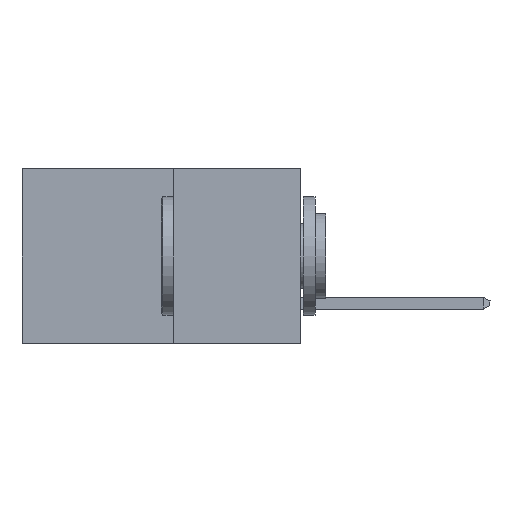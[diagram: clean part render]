
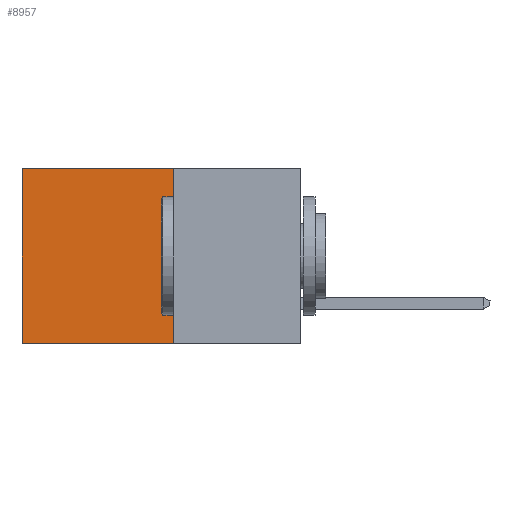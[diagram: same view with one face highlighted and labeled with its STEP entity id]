
A CAD part, left-side view. The second image highlights one B-rep face of the part: STEP entity #8957.
In plain terms, the highlighted planar face has unit normal (-1, 0, 0).
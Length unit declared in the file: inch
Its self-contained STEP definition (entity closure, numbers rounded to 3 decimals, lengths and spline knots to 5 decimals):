
#61 = DIRECTION ( 'NONE',  ( 0., 0., -1. ) ) ;
#277 = CARTESIAN_POINT ( 'NONE',  ( 0.277, 0.59, -0.37 ) ) ;
#742 = EDGE_CURVE ( 'NONE', #8258, #9761, #7570, .T. ) ;
#885 = VECTOR ( 'NONE', #9898, 39.37008 ) ;
#2370 = CARTESIAN_POINT ( 'NONE',  ( 0.277, 0.27, 0. ) ) ;
#2500 = CARTESIAN_POINT ( 'NONE',  ( 0.277, 0.27, -0.37 ) ) ;
#2639 = PLANE ( 'NONE',  #7540 ) ;
#3085 = VECTOR ( 'NONE', #8070, 39.37008 ) ;
#3490 = DIRECTION ( 'NONE',  ( 1., 0., 0. ) ) ;
#3714 = EDGE_CURVE ( 'NONE', #6732, #6350, #4821, .T. ) ;
#3799 = EDGE_LOOP ( 'NONE', ( #10205, #10241, #10270, #10334 ) ) ;
#4128 = EDGE_CURVE ( 'NONE', #8258, #6732, #5062, .T. ) ;
#4821 = LINE ( 'NONE', #277, #8914 ) ;
#5062 = LINE ( 'NONE', #8074, #3085 ) ;
#5305 = CARTESIAN_POINT ( 'NONE',  ( 0.277, 0.27, -0.37 ) ) ;
#6109 = EDGE_CURVE ( 'NONE', #9761, #6350, #7330, .T. ) ;
#6156 = DIRECTION ( 'NONE',  ( 0., 1., 0. ) ) ;
#6166 = CARTESIAN_POINT ( 'NONE',  ( 0.277, 0.59, -0.37 ) ) ;
#6350 = VERTEX_POINT ( 'NONE', #6166 ) ;
#6732 = VERTEX_POINT ( 'NONE', #10495 ) ;
#7316 = CARTESIAN_POINT ( 'NONE',  ( 0.277, 0.27, -0.37 ) ) ;
#7330 = LINE ( 'NONE', #5305, #9215 ) ;
#7530 = FACE_OUTER_BOUND ( 'NONE', #3799, .T. ) ;
#7540 = AXIS2_PLACEMENT_3D ( 'NONE', #8450, #3490, #9220 ) ;
#7570 = LINE ( 'NONE', #2500, #885 ) ;
#8070 = DIRECTION ( 'NONE',  ( 0., 1., 0. ) ) ;
#8074 = CARTESIAN_POINT ( 'NONE',  ( 0.277, 0.27, 0. ) ) ;
#8258 = VERTEX_POINT ( 'NONE', #2370 ) ;
#8450 = CARTESIAN_POINT ( 'NONE',  ( 0.277, 0.27, -0.37 ) ) ;
#8914 = VECTOR ( 'NONE', #61, 39.37008 ) ;
#8957 = ADVANCED_FACE ( 'NONE', ( #7530 ), #2639, .F. ) ;
#9215 = VECTOR ( 'NONE', #6156, 39.37008 ) ;
#9220 = DIRECTION ( 'NONE',  ( 0., 0., -1. ) ) ;
#9761 = VERTEX_POINT ( 'NONE', #7316 ) ;
#9898 = DIRECTION ( 'NONE',  ( 0., 0., -1. ) ) ;
#10205 = ORIENTED_EDGE ( 'NONE', *, *, #3714, .T. ) ;
#10241 = ORIENTED_EDGE ( 'NONE', *, *, #6109, .F. ) ;
#10270 = ORIENTED_EDGE ( 'NONE', *, *, #742, .F. ) ;
#10334 = ORIENTED_EDGE ( 'NONE', *, *, #4128, .T. ) ;
#10495 = CARTESIAN_POINT ( 'NONE',  ( 0.277, 0.59, 0. ) ) ;
